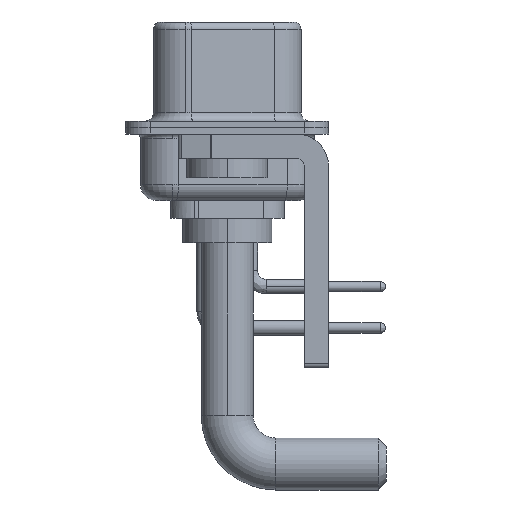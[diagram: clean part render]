
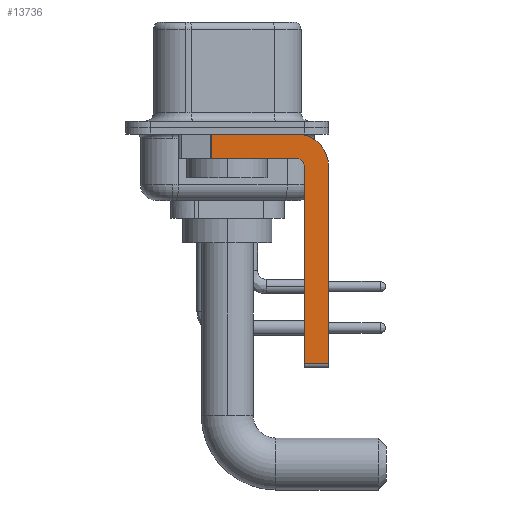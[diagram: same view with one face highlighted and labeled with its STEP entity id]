
A CAD part, left-side view. The second image highlights one B-rep face of the part: STEP entity #13736.
In plain terms, the highlighted planar face has unit normal (-1, 0, 0).
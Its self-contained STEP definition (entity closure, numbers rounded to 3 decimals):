
#153 = EDGE_CURVE ( 'NONE', #1132, #2296, #8430, .T. ) ;
#167 = CARTESIAN_POINT ( 'NONE',  ( -2.9, 0.978, -1.9 ) ) ;
#765 = ORIENTED_EDGE ( 'NONE', *, *, #153, .F. ) ;
#948 = ORIENTED_EDGE ( 'NONE', *, *, #13793, .F. ) ;
#1132 = VERTEX_POINT ( 'NONE', #6067 ) ;
#1430 = EDGE_CURVE ( 'NONE', #9857, #15305, #11051, .T. ) ;
#1631 = EDGE_CURVE ( 'NONE', #5833, #3483, #15377, .T. ) ;
#2296 = VERTEX_POINT ( 'NONE', #8497 ) ;
#2533 = VECTOR ( 'NONE', #11174, 1000. ) ;
#2977 = CARTESIAN_POINT ( 'NONE',  ( -2.9, -6.25, -14.55 ) ) ;
#3483 = VERTEX_POINT ( 'NONE', #13488 ) ;
#3955 = CARTESIAN_POINT ( 'NONE',  ( -2.9, -4.25, -2.4 ) ) ;
#4123 = DIRECTION ( 'NONE',  ( 0., 0., -1. ) ) ;
#4506 = VECTOR ( 'NONE', #22891, 1000. ) ;
#4652 = LINE ( 'NONE', #8034, #20058 ) ;
#5535 = CARTESIAN_POINT ( 'NONE',  ( -2.9, -4.75, -14.8 ) ) ;
#5833 = VERTEX_POINT ( 'NONE', #7018 ) ;
#5910 = CARTESIAN_POINT ( 'NONE',  ( -2.9, -4.25, -2.4 ) ) ;
#6067 = CARTESIAN_POINT ( 'NONE',  ( -2.9, -4.25, -1.9 ) ) ;
#6074 = PLANE ( 'NONE',  #13674 ) ;
#6611 = AXIS2_PLACEMENT_3D ( 'NONE', #5910, #17595, #9662 ) ;
#6857 = ORIENTED_EDGE ( 'NONE', *, *, #1430, .T. ) ;
#7018 = CARTESIAN_POINT ( 'NONE',  ( -2.9, -4.25, -0.4 ) ) ;
#7575 = DIRECTION ( 'NONE',  ( 1., 0., 0. ) ) ;
#8034 = CARTESIAN_POINT ( 'NONE',  ( -2.9, 3., -0.4 ) ) ;
#8430 = LINE ( 'NONE', #18246, #23808 ) ;
#8497 = CARTESIAN_POINT ( 'NONE',  ( -2.9, 0.978, -1.9 ) ) ;
#8570 = ORIENTED_EDGE ( 'NONE', *, *, #14250, .F. ) ;
#9662 = DIRECTION ( 'NONE',  ( 0., 0., -1. ) ) ;
#9857 = VERTEX_POINT ( 'NONE', #18148 ) ;
#9931 = CARTESIAN_POINT ( 'NONE',  ( -2.9, -4.75, -2.4 ) ) ;
#11051 = LINE ( 'NONE', #13158, #2533 ) ;
#11174 = DIRECTION ( 'NONE',  ( 0., -1., 0. ) ) ;
#11403 = VECTOR ( 'NONE', #4123, 1000. ) ;
#13158 = CARTESIAN_POINT ( 'NONE',  ( -2.9, -4.25, -14.55 ) ) ;
#13488 = CARTESIAN_POINT ( 'NONE',  ( -2.9, -6.25, -2.4 ) ) ;
#13674 = AXIS2_PLACEMENT_3D ( 'NONE', #17387, #7575, #15296 ) ;
#13736 = ADVANCED_FACE ( 'NONE', ( #21102 ), #6074, .F. ) ;
#13793 = EDGE_CURVE ( 'NONE', #24099, #1132, #23145, .T. ) ;
#13908 = DIRECTION ( 'NONE',  ( 0., 1., 0. ) ) ;
#14250 = EDGE_CURVE ( 'NONE', #24186, #5833, #4652, .T. ) ;
#14756 = CARTESIAN_POINT ( 'NONE',  ( -2.9, -6.25, -2.4 ) ) ;
#15296 = DIRECTION ( 'NONE',  ( 0., 0., -1. ) ) ;
#15305 = VERTEX_POINT ( 'NONE', #2977 ) ;
#15377 = CIRCLE ( 'NONE', #6611, 2. ) ;
#15819 = EDGE_CURVE ( 'NONE', #9857, #24099, #22533, .T. ) ;
#16619 = LINE ( 'NONE', #14756, #24091 ) ;
#16788 = ORIENTED_EDGE ( 'NONE', *, *, #15819, .F. ) ;
#17387 = CARTESIAN_POINT ( 'NONE',  ( -2.9, -4.25, -2.4 ) ) ;
#17595 = DIRECTION ( 'NONE',  ( 1., 0., 0. ) ) ;
#18061 = ORIENTED_EDGE ( 'NONE', *, *, #18560, .T. ) ;
#18148 = CARTESIAN_POINT ( 'NONE',  ( -2.9, -4.75, -14.55 ) ) ;
#18246 = CARTESIAN_POINT ( 'NONE',  ( -2.9, -4.25, -1.9 ) ) ;
#18419 = AXIS2_PLACEMENT_3D ( 'NONE', #3955, #19124, #19362 ) ;
#18560 = EDGE_CURVE ( 'NONE', #24186, #2296, #19052, .T. ) ;
#18992 = ORIENTED_EDGE ( 'NONE', *, *, #1631, .F. ) ;
#19052 = LINE ( 'NONE', #167, #11403 ) ;
#19124 = DIRECTION ( 'NONE',  ( -1., 0., 0. ) ) ;
#19362 = DIRECTION ( 'NONE',  ( 0., 0., 1. ) ) ;
#20058 = VECTOR ( 'NONE', #23161, 1000. ) ;
#21079 = EDGE_CURVE ( 'NONE', #3483, #15305, #16619, .T. ) ;
#21102 = FACE_OUTER_BOUND ( 'NONE', #21391, .T. ) ;
#21391 = EDGE_LOOP ( 'NONE', ( #8570, #18061, #765, #948, #16788, #6857, #23825, #18992 ) ) ;
#21692 = CARTESIAN_POINT ( 'NONE',  ( -2.9, 0.978, -0.4 ) ) ;
#22290 = DIRECTION ( 'NONE',  ( 0., 0., -1. ) ) ;
#22533 = LINE ( 'NONE', #5535, #4506 ) ;
#22891 = DIRECTION ( 'NONE',  ( 0., 0., 1. ) ) ;
#23145 = CIRCLE ( 'NONE', #18419, 0.5 ) ;
#23161 = DIRECTION ( 'NONE',  ( 0., -1., 0. ) ) ;
#23808 = VECTOR ( 'NONE', #13908, 1000. ) ;
#23825 = ORIENTED_EDGE ( 'NONE', *, *, #21079, .F. ) ;
#24091 = VECTOR ( 'NONE', #22290, 1000. ) ;
#24099 = VERTEX_POINT ( 'NONE', #9931 ) ;
#24186 = VERTEX_POINT ( 'NONE', #21692 ) ;
